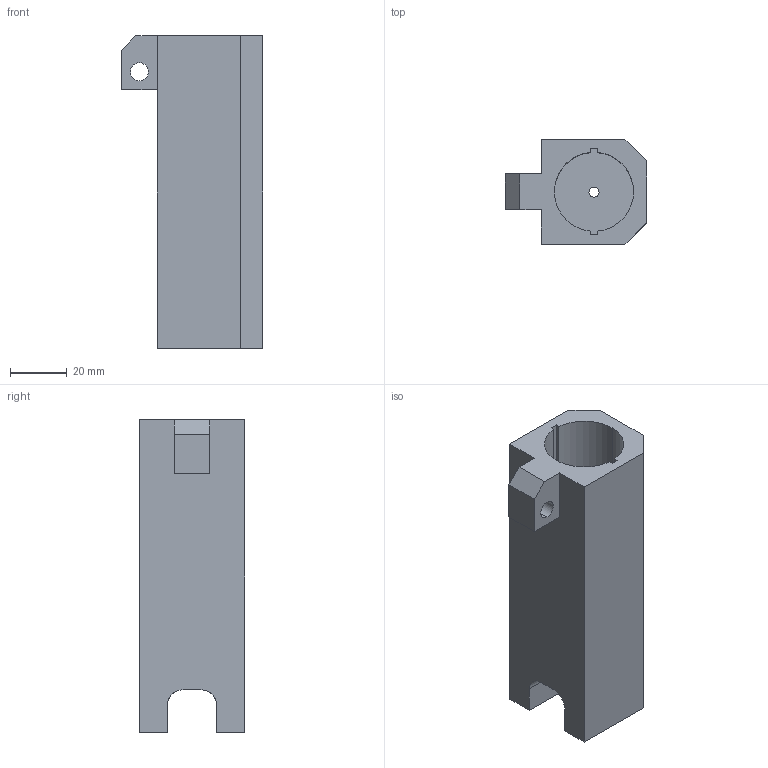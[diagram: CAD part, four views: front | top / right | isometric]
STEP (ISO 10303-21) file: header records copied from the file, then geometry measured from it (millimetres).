
FILE_DESCRIPTION (( 'STEP AP214' ), '1' );
FILE_NAME ('sec_2.STEP', '2013-10-23T01:31:39', ( '' ), ( '' ), 'SwSTEP 2.0', 'SolidWorks 2013', '' );
FILE_SCHEMA (( 'AUTOMOTIVE_DESIGN' ));
Length unit declared in the file: inch
Products named in the file (1): sec_2
Bounding box: 49.78 x 37.08 x 110.2 mm (x, y, z)
Volume: 82892.4 mm3; surface area: 27723.3 mm2
Topology: 1 solids, 1 shells, 44 faces, 125 edges, 83 vertices
Faces by surface type: plane 33, cylinder 11
Entity records: 1476 total; most frequent: CARTESIAN_POINT 262, ORIENTED_EDGE 250, DIRECTION 235, EDGE_CURVE 125, LINE 99, VECTOR 99, VERTEX_POINT 83, AXIS2_PLACEMENT_3D 68
